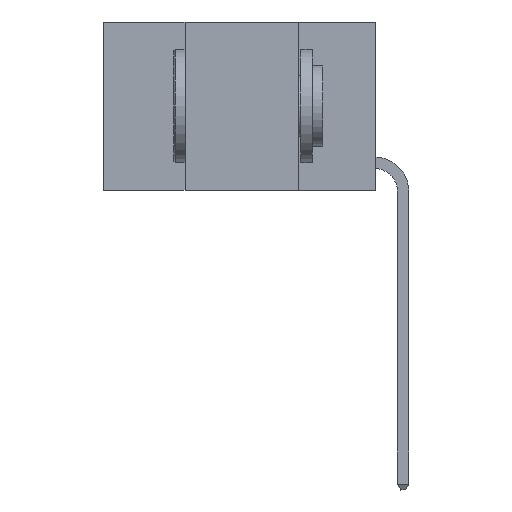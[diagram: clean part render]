
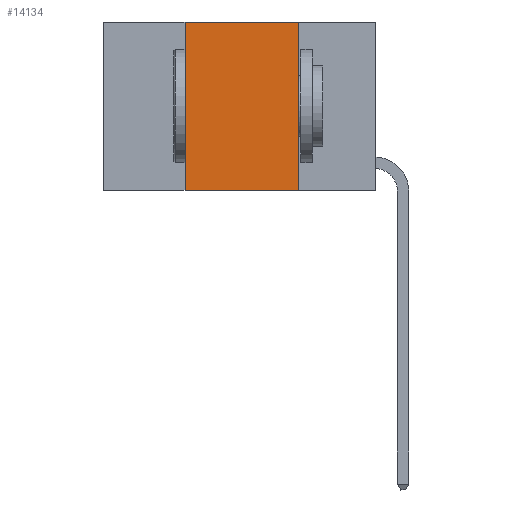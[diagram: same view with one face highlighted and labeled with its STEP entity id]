
A CAD part, left-side view. The second image highlights one B-rep face of the part: STEP entity #14134.
In plain terms, the highlighted planar face has unit normal (-1, 0, 0).
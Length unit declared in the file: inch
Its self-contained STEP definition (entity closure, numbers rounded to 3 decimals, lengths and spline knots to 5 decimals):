
#289 = LINE ( 'NONE', #6167, #14587 ) ;
#507 = CARTESIAN_POINT ( 'NONE',  ( 0., 0.42, -0.37 ) ) ;
#927 = FACE_OUTER_BOUND ( 'NONE', #14196, .T. ) ;
#1689 = VECTOR ( 'NONE', #18225, 39.37008 ) ;
#1768 = LINE ( 'NONE', #10836, #3236 ) ;
#1928 = ORIENTED_EDGE ( 'NONE', *, *, #7336, .F. ) ;
#2183 = LINE ( 'NONE', #6428, #1689 ) ;
#2378 = CARTESIAN_POINT ( 'NONE',  ( 0., 0.6, -0.37 ) ) ;
#3236 = VECTOR ( 'NONE', #4846, 39.37008 ) ;
#3356 = ORIENTED_EDGE ( 'NONE', *, *, #19020, .T. ) ;
#3924 = DIRECTION ( 'NONE',  ( 1., 0., 0. ) ) ;
#3944 = DIRECTION ( 'NONE',  ( 0., 0., -1. ) ) ;
#4846 = DIRECTION ( 'NONE',  ( 0., 0., 1. ) ) ;
#5251 = EDGE_CURVE ( 'NONE', #8519, #14363, #2183, .T. ) ;
#6167 = CARTESIAN_POINT ( 'NONE',  ( 0., 0.17, 0. ) ) ;
#6428 = CARTESIAN_POINT ( 'NONE',  ( 0., 0.6, 0. ) ) ;
#6820 = CARTESIAN_POINT ( 'NONE',  ( 0., 0.6, 0. ) ) ;
#7053 = CARTESIAN_POINT ( 'NONE',  ( 0., 0.42, 0. ) ) ;
#7336 = EDGE_CURVE ( 'NONE', #14764, #8519, #1768, .T. ) ;
#7513 = VECTOR ( 'NONE', #14061, 39.37008 ) ;
#8519 = VERTEX_POINT ( 'NONE', #7053 ) ;
#10836 = CARTESIAN_POINT ( 'NONE',  ( 0., 0.42, 0. ) ) ;
#11378 = AXIS2_PLACEMENT_3D ( 'NONE', #6820, #3924, #18705 ) ;
#12796 = PLANE ( 'NONE',  #11378 ) ;
#14061 = DIRECTION ( 'NONE',  ( 0., -1., 0. ) ) ;
#14067 = ORIENTED_EDGE ( 'NONE', *, *, #18483, .F. ) ;
#14134 = ADVANCED_FACE ( 'NONE', ( #927 ), #12796, .F. ) ;
#14196 = EDGE_LOOP ( 'NONE', ( #14067, #14927, #1928, #3356 ) ) ;
#14363 = VERTEX_POINT ( 'NONE', #15209 ) ;
#14587 = VECTOR ( 'NONE', #3944, 39.37008 ) ;
#14675 = CARTESIAN_POINT ( 'NONE',  ( 0., 0.17, -0.37 ) ) ;
#14764 = VERTEX_POINT ( 'NONE', #507 ) ;
#14927 = ORIENTED_EDGE ( 'NONE', *, *, #5251, .F. ) ;
#15209 = CARTESIAN_POINT ( 'NONE',  ( 0., 0.17, 0. ) ) ;
#15422 = LINE ( 'NONE', #2378, #7513 ) ;
#18225 = DIRECTION ( 'NONE',  ( 0., -1., 0. ) ) ;
#18237 = VERTEX_POINT ( 'NONE', #14675 ) ;
#18483 = EDGE_CURVE ( 'NONE', #14363, #18237, #289, .T. ) ;
#18705 = DIRECTION ( 'NONE',  ( 0., 0., -1. ) ) ;
#19020 = EDGE_CURVE ( 'NONE', #14764, #18237, #15422, .T. ) ;
